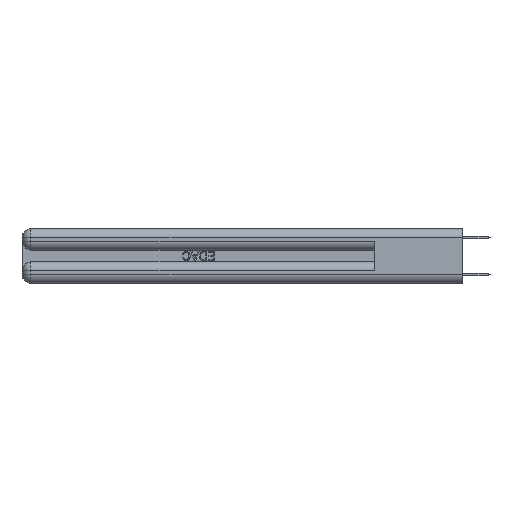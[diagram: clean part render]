
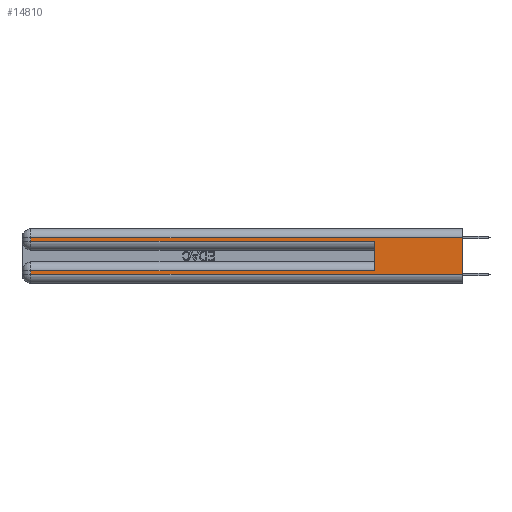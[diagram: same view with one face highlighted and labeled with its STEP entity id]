
A CAD part, left-side view. The second image highlights one B-rep face of the part: STEP entity #14810.
In plain terms, the highlighted planar face has unit normal (-1, 0, 0).
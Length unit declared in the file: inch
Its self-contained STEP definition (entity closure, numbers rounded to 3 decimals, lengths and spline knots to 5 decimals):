
#23 = ORIENTED_EDGE ( 'NONE', *, *, #28517, .F. ) ;
#748 = ORIENTED_EDGE ( 'NONE', *, *, #15523, .T. ) ;
#5234 = ORIENTED_EDGE ( 'NONE', *, *, #30919, .T. ) ;
#5426 = VERTEX_POINT ( 'NONE', #24558 ) ;
#5473 = LINE ( 'NONE', #8247, #24635 ) ;
#5735 = LINE ( 'NONE', #29117, #30711 ) ;
#5885 = CARTESIAN_POINT ( 'NONE',  ( 0., 0.6, 0.085 ) ) ;
#6251 = LINE ( 'NONE', #16971, #30747 ) ;
#6341 = LINE ( 'NONE', #16896, #32820 ) ;
#6839 = ORIENTED_EDGE ( 'NONE', *, *, #18250, .F. ) ;
#7054 = VERTEX_POINT ( 'NONE', #8096 ) ;
#7383 = PLANE ( 'NONE',  #13962 ) ;
#8057 = CARTESIAN_POINT ( 'NONE',  ( 0., 0., 0.37 ) ) ;
#8073 = EDGE_CURVE ( 'NONE', #5426, #7054, #5473, .T. ) ;
#8096 = CARTESIAN_POINT ( 'NONE',  ( 0., 2.94, 0.06 ) ) ;
#8247 = CARTESIAN_POINT ( 'NONE',  ( 0., 2.94, 0.37 ) ) ;
#8347 = ORIENTED_EDGE ( 'NONE', *, *, #31027, .T. ) ;
#10136 = DIRECTION ( 'NONE',  ( 0., 0., -1. ) ) ;
#12263 = VECTOR ( 'NONE', #25799, 39.37008 ) ;
#12525 = ORIENTED_EDGE ( 'NONE', *, *, #13781, .T. ) ;
#12653 = LINE ( 'NONE', #28241, #12263 ) ;
#12658 = VERTEX_POINT ( 'NONE', #5885 ) ;
#12712 = CARTESIAN_POINT ( 'NONE',  ( 0., 0., 0.06 ) ) ;
#13366 = VERTEX_POINT ( 'NONE', #16906 ) ;
#13741 = DIRECTION ( 'NONE',  ( 0., 1., 0. ) ) ;
#13781 = EDGE_CURVE ( 'NONE', #23517, #13366, #12653, .T. ) ;
#13906 = LINE ( 'NONE', #31761, #30881 ) ;
#13962 = AXIS2_PLACEMENT_3D ( 'NONE', #8057, #25727, #10136 ) ;
#14394 = EDGE_LOOP ( 'NONE', ( #6839, #8347, #23557, #12525, #23, #748, #16535, #5234 ) ) ;
#14723 = LINE ( 'NONE', #31003, #22548 ) ;
#14810 = ADVANCED_FACE ( 'NONE', ( #18109 ), #7383, .F. ) ;
#15280 = CARTESIAN_POINT ( 'NONE',  ( 0., 0., 0.06 ) ) ;
#15523 = EDGE_CURVE ( 'NONE', #12658, #5426, #6341, .T. ) ;
#16535 = ORIENTED_EDGE ( 'NONE', *, *, #8073, .T. ) ;
#16896 = CARTESIAN_POINT ( 'NONE',  ( 0., 0., 0.085 ) ) ;
#16906 = CARTESIAN_POINT ( 'NONE',  ( 0., 0.6, 0.285 ) ) ;
#16958 = DIRECTION ( 'NONE',  ( 0., 0., 1. ) ) ;
#16971 = CARTESIAN_POINT ( 'NONE',  ( 0., 0., 0.37 ) ) ;
#17145 = DIRECTION ( 'NONE',  ( 0., 0., -1. ) ) ;
#18109 = FACE_OUTER_BOUND ( 'NONE', #14394, .T. ) ;
#18125 = CARTESIAN_POINT ( 'NONE',  ( 0., 0., 0.31 ) ) ;
#18250 = EDGE_CURVE ( 'NONE', #31626, #31411, #6251, .T. ) ;
#19068 = CARTESIAN_POINT ( 'NONE',  ( 0., 2.94, 0.31 ) ) ;
#21266 = CARTESIAN_POINT ( 'NONE',  ( 0., 2.94, 0.285 ) ) ;
#21310 = DIRECTION ( 'NONE',  ( 0., 0., -1. ) ) ;
#21567 = DIRECTION ( 'NONE',  ( 0., 0., -1. ) ) ;
#22548 = VECTOR ( 'NONE', #16958, 39.37008 ) ;
#23517 = VERTEX_POINT ( 'NONE', #21266 ) ;
#23557 = ORIENTED_EDGE ( 'NONE', *, *, #25569, .T. ) ;
#24558 = CARTESIAN_POINT ( 'NONE',  ( 0., 2.94, 0.085 ) ) ;
#24635 = VECTOR ( 'NONE', #21567, 39.37008 ) ;
#25569 = EDGE_CURVE ( 'NONE', #25761, #23517, #5735, .T. ) ;
#25727 = DIRECTION ( 'NONE',  ( 1., 0., 0. ) ) ;
#25761 = VERTEX_POINT ( 'NONE', #19068 ) ;
#25799 = DIRECTION ( 'NONE',  ( 0., -1., 0. ) ) ;
#27626 = DIRECTION ( 'NONE',  ( 0., 1., 0. ) ) ;
#28241 = CARTESIAN_POINT ( 'NONE',  ( 0., 0., 0.285 ) ) ;
#28517 = EDGE_CURVE ( 'NONE', #12658, #13366, #14723, .T. ) ;
#29117 = CARTESIAN_POINT ( 'NONE',  ( 0., 2.94, 0.37 ) ) ;
#30711 = VECTOR ( 'NONE', #21310, 39.37008 ) ;
#30747 = VECTOR ( 'NONE', #17145, 39.37008 ) ;
#30881 = VECTOR ( 'NONE', #13741, 39.37008 ) ;
#30919 = EDGE_CURVE ( 'NONE', #7054, #31411, #33513, .T. ) ;
#31003 = CARTESIAN_POINT ( 'NONE',  ( 0., 0.6, 0.145 ) ) ;
#31027 = EDGE_CURVE ( 'NONE', #31626, #25761, #13906, .T. ) ;
#31411 = VERTEX_POINT ( 'NONE', #15280 ) ;
#31626 = VERTEX_POINT ( 'NONE', #18125 ) ;
#31761 = CARTESIAN_POINT ( 'NONE',  ( 0., 0., 0.31 ) ) ;
#32528 = VECTOR ( 'NONE', #34018, 39.37008 ) ;
#32820 = VECTOR ( 'NONE', #27626, 39.37008 ) ;
#33513 = LINE ( 'NONE', #12712, #32528 ) ;
#34018 = DIRECTION ( 'NONE',  ( 0., -1., 0. ) ) ;
